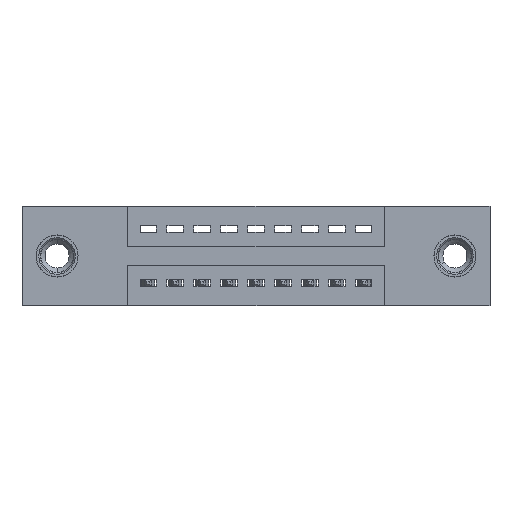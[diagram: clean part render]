
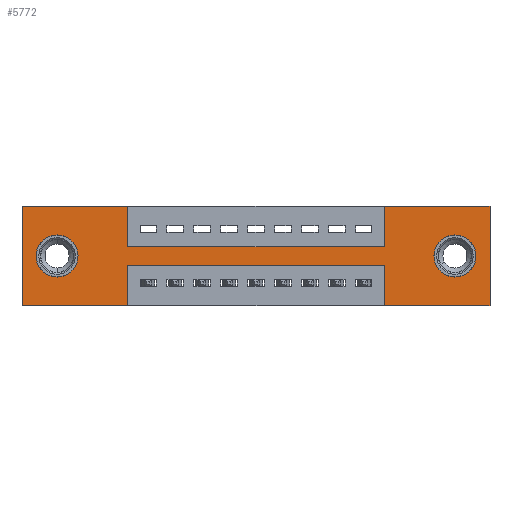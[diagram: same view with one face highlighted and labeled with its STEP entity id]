
A CAD part, front view. The second image highlights one B-rep face of the part: STEP entity #5772.
In plain terms, the highlighted planar face has unit normal (0, -1, 0).
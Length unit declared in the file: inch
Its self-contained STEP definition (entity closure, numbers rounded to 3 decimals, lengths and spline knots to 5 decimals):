
#291 = VERTEX_POINT ( 'NONE', #11541 ) ;
#350 = ORIENTED_EDGE ( 'NONE', *, *, #7089, .F. ) ;
#595 = ORIENTED_EDGE ( 'NONE', *, *, #1682, .F. ) ;
#609 = AXIS2_PLACEMENT_3D ( 'NONE', #12363, #6774, #968 ) ;
#776 = ORIENTED_EDGE ( 'NONE', *, *, #9528, .F. ) ;
#789 = CARTESIAN_POINT ( 'NONE',  ( 0., 0., 0. ) ) ;
#835 = ORIENTED_EDGE ( 'NONE', *, *, #6167, .T. ) ;
#839 = LINE ( 'NONE', #3806, #8551 ) ;
#843 = VECTOR ( 'NONE', #8535, 39.37008 ) ;
#883 = CARTESIAN_POINT ( 'NONE',  ( 1.3425, 0., 0. ) ) ;
#905 = LINE ( 'NONE', #2048, #5767 ) ;
#967 = EDGE_CURVE ( 'NONE', #3909, #5645, #2659, .T. ) ;
#968 = DIRECTION ( 'NONE',  ( 0., 0., 1. ) ) ;
#1172 = DIRECTION ( 'NONE',  ( 0., 0., -1. ) ) ;
#1248 = AXIS2_PLACEMENT_3D ( 'NONE', #11172, #5536, #12098 ) ;
#1309 = VERTEX_POINT ( 'NONE', #11852 ) ;
#1364 = CARTESIAN_POINT ( 'NONE',  ( 1.3425, 0., -0.37 ) ) ;
#1485 = VERTEX_POINT ( 'NONE', #883 ) ;
#1540 = EDGE_CURVE ( 'NONE', #4583, #1983, #10960, .T. ) ;
#1682 = EDGE_CURVE ( 'NONE', #1485, #10315, #11670, .T. ) ;
#1812 = VECTOR ( 'NONE', #2755, 39.37008 ) ;
#1960 = CARTESIAN_POINT ( 'NONE',  ( 0.3925, 0., 0. ) ) ;
#1983 = VERTEX_POINT ( 'NONE', #8934 ) ;
#2048 = CARTESIAN_POINT ( 'NONE',  ( 0.3925, 0., -0.15 ) ) ;
#2102 = VECTOR ( 'NONE', #9340, 39.37008 ) ;
#2384 = ORIENTED_EDGE ( 'NONE', *, *, #7300, .T. ) ;
#2472 = CARTESIAN_POINT ( 'NONE',  ( 0.3925, 0., -0.22 ) ) ;
#2659 = CIRCLE ( 'NONE', #7016, 0.078 ) ;
#2755 = DIRECTION ( 'NONE',  ( -1., 0., 0. ) ) ;
#2820 = EDGE_CURVE ( 'NONE', #4126, #1309, #3379, .T. ) ;
#2855 = LINE ( 'NONE', #1960, #7664 ) ;
#2918 = CARTESIAN_POINT ( 'NONE',  ( 0.13, 0., -0.107 ) ) ;
#2984 = EDGE_CURVE ( 'NONE', #9072, #1485, #9177, .T. ) ;
#3079 = VERTEX_POINT ( 'NONE', #8662 ) ;
#3239 = ORIENTED_EDGE ( 'NONE', *, *, #5587, .F. ) ;
#3243 = VERTEX_POINT ( 'NONE', #1364 ) ;
#3330 = DIRECTION ( 'NONE',  ( 0., 0., -1. ) ) ;
#3379 = CIRCLE ( 'NONE', #7757, 0.078 ) ;
#3417 = VECTOR ( 'NONE', #7366, 39.37008 ) ;
#3422 = EDGE_CURVE ( 'NONE', #10061, #3079, #9454, .T. ) ;
#3432 = CIRCLE ( 'NONE', #1248, 0.078 ) ;
#3484 = LINE ( 'NONE', #11287, #843 ) ;
#3499 = EDGE_CURVE ( 'NONE', #3079, #291, #8580, .T. ) ;
#3501 = DIRECTION ( 'NONE',  ( 0., 1., 0. ) ) ;
#3519 = VECTOR ( 'NONE', #7538, 39.37008 ) ;
#3806 = CARTESIAN_POINT ( 'NONE',  ( 0., 0., -0.37 ) ) ;
#3848 = DIRECTION ( 'NONE',  ( 0., 0., -1. ) ) ;
#3909 = VERTEX_POINT ( 'NONE', #9100 ) ;
#3915 = FACE_BOUND ( 'NONE', #11720, .T. ) ;
#3995 = DIRECTION ( 'NONE',  ( 1., 0., 0. ) ) ;
#4126 = VERTEX_POINT ( 'NONE', #12198 ) ;
#4287 = CARTESIAN_POINT ( 'NONE',  ( 1.735, 0., 0. ) ) ;
#4409 = VECTOR ( 'NONE', #9259, 39.37008 ) ;
#4583 = VERTEX_POINT ( 'NONE', #5063 ) ;
#4952 = ORIENTED_EDGE ( 'NONE', *, *, #2820, .T. ) ;
#5037 = PLANE ( 'NONE',  #9493 ) ;
#5063 = CARTESIAN_POINT ( 'NONE',  ( 1.3425, 0., -0.22 ) ) ;
#5075 = ORIENTED_EDGE ( 'NONE', *, *, #2984, .F. ) ;
#5178 = DIRECTION ( 'NONE',  ( 0., 1., 0. ) ) ;
#5480 = CARTESIAN_POINT ( 'NONE',  ( 1.3425, 0., -0.15 ) ) ;
#5482 = EDGE_CURVE ( 'NONE', #1983, #12427, #7516, .T. ) ;
#5533 = CARTESIAN_POINT ( 'NONE',  ( 0.3925, 0., -0.37 ) ) ;
#5536 = DIRECTION ( 'NONE',  ( 0., 1., 0. ) ) ;
#5587 = EDGE_CURVE ( 'NONE', #12329, #3243, #839, .T. ) ;
#5643 = EDGE_CURVE ( 'NONE', #291, #11051, #2855, .T. ) ;
#5645 = VERTEX_POINT ( 'NONE', #2918 ) ;
#5767 = VECTOR ( 'NONE', #3995, 39.37008 ) ;
#5772 = ADVANCED_FACE ( 'NONE', ( #11153, #3915, #6476 ), #5037, .T. ) ;
#5943 = CARTESIAN_POINT ( 'NONE',  ( 0., 0., -0.37 ) ) ;
#6167 = EDGE_CURVE ( 'NONE', #5645, #3909, #6460, .T. ) ;
#6460 = CIRCLE ( 'NONE', #609, 0.078 ) ;
#6476 = FACE_OUTER_BOUND ( 'NONE', #9864, .T. ) ;
#6579 = CARTESIAN_POINT ( 'NONE',  ( 0., 0., 0. ) ) ;
#6580 = ORIENTED_EDGE ( 'NONE', *, *, #3422, .F. ) ;
#6774 = DIRECTION ( 'NONE',  ( 0., 1., 0. ) ) ;
#6942 = DIRECTION ( 'NONE',  ( 0., -1., 0. ) ) ;
#7016 = AXIS2_PLACEMENT_3D ( 'NONE', #11821, #5178, #11853 ) ;
#7089 = EDGE_CURVE ( 'NONE', #10315, #12329, #8656, .T. ) ;
#7236 = CARTESIAN_POINT ( 'NONE',  ( 1.735, 0., -0.37 ) ) ;
#7300 = EDGE_CURVE ( 'NONE', #1309, #4126, #3432, .T. ) ;
#7366 = DIRECTION ( 'NONE',  ( -1., 0., 0. ) ) ;
#7516 = LINE ( 'NONE', #5533, #2102 ) ;
#7538 = DIRECTION ( 'NONE',  ( 1., 0., 0. ) ) ;
#7572 = DIRECTION ( 'NONE',  ( 1., 0., 0. ) ) ;
#7664 = VECTOR ( 'NONE', #3848, 39.37008 ) ;
#7757 = AXIS2_PLACEMENT_3D ( 'NONE', #9188, #3501, #10126 ) ;
#8372 = CARTESIAN_POINT ( 'NONE',  ( 0., 0., 0. ) ) ;
#8399 = EDGE_LOOP ( 'NONE', ( #2384, #4952 ) ) ;
#8501 = DIRECTION ( 'NONE',  ( 0., 0., 1. ) ) ;
#8535 = DIRECTION ( 'NONE',  ( 0., 0., 1. ) ) ;
#8551 = VECTOR ( 'NONE', #10426, 39.37008 ) ;
#8580 = LINE ( 'NONE', #6579, #3519 ) ;
#8607 = CARTESIAN_POINT ( 'NONE',  ( 0., 0., -0.37 ) ) ;
#8656 = LINE ( 'NONE', #4287, #11125 ) ;
#8662 = CARTESIAN_POINT ( 'NONE',  ( 0., 0., 0. ) ) ;
#8720 = ORIENTED_EDGE ( 'NONE', *, *, #11927, .F. ) ;
#8817 = CARTESIAN_POINT ( 'NONE',  ( 1.735, 0., 0. ) ) ;
#8854 = LINE ( 'NONE', #9425, #1812 ) ;
#8896 = VECTOR ( 'NONE', #8501, 39.37008 ) ;
#8934 = CARTESIAN_POINT ( 'NONE',  ( 0.3925, 0., -0.22 ) ) ;
#9072 = VERTEX_POINT ( 'NONE', #5480 ) ;
#9100 = CARTESIAN_POINT ( 'NONE',  ( 0.13, 0., -0.263 ) ) ;
#9129 = CARTESIAN_POINT ( 'NONE',  ( 0.3925, 0., -0.15 ) ) ;
#9177 = LINE ( 'NONE', #11247, #8896 ) ;
#9188 = CARTESIAN_POINT ( 'NONE',  ( 1.605, 0., -0.185 ) ) ;
#9259 = DIRECTION ( 'NONE',  ( 0., 0., 1. ) ) ;
#9340 = DIRECTION ( 'NONE',  ( 0., 0., -1. ) ) ;
#9425 = CARTESIAN_POINT ( 'NONE',  ( 0., 0., -0.37 ) ) ;
#9454 = LINE ( 'NONE', #8372, #4409 ) ;
#9493 = AXIS2_PLACEMENT_3D ( 'NONE', #5943, #6942, #1172 ) ;
#9528 = EDGE_CURVE ( 'NONE', #11051, #9072, #905, .T. ) ;
#9847 = ORIENTED_EDGE ( 'NONE', *, *, #11904, .F. ) ;
#9864 = EDGE_LOOP ( 'NONE', ( #11076, #10037, #8720, #3239, #350, #595, #5075, #776, #11135, #11564, #6580, #9847 ) ) ;
#10003 = ORIENTED_EDGE ( 'NONE', *, *, #967, .T. ) ;
#10037 = ORIENTED_EDGE ( 'NONE', *, *, #1540, .F. ) ;
#10061 = VERTEX_POINT ( 'NONE', #8607 ) ;
#10126 = DIRECTION ( 'NONE',  ( 0., 0., -1. ) ) ;
#10221 = CARTESIAN_POINT ( 'NONE',  ( 0.3925, 0., -0.37 ) ) ;
#10315 = VERTEX_POINT ( 'NONE', #8817 ) ;
#10426 = DIRECTION ( 'NONE',  ( -1., 0., 0. ) ) ;
#10960 = LINE ( 'NONE', #2472, #3417 ) ;
#11051 = VERTEX_POINT ( 'NONE', #9129 ) ;
#11076 = ORIENTED_EDGE ( 'NONE', *, *, #5482, .F. ) ;
#11125 = VECTOR ( 'NONE', #3330, 39.37008 ) ;
#11135 = ORIENTED_EDGE ( 'NONE', *, *, #5643, .F. ) ;
#11153 = FACE_BOUND ( 'NONE', #8399, .T. ) ;
#11172 = CARTESIAN_POINT ( 'NONE',  ( 1.605, 0., -0.185 ) ) ;
#11247 = CARTESIAN_POINT ( 'NONE',  ( 1.3425, 0., 0. ) ) ;
#11287 = CARTESIAN_POINT ( 'NONE',  ( 1.3425, 0., -0.37 ) ) ;
#11541 = CARTESIAN_POINT ( 'NONE',  ( 0.3925, 0., 0. ) ) ;
#11564 = ORIENTED_EDGE ( 'NONE', *, *, #3499, .F. ) ;
#11670 = LINE ( 'NONE', #789, #11966 ) ;
#11720 = EDGE_LOOP ( 'NONE', ( #835, #10003 ) ) ;
#11821 = CARTESIAN_POINT ( 'NONE',  ( 0.13, 0., -0.185 ) ) ;
#11852 = CARTESIAN_POINT ( 'NONE',  ( 1.605, 0., -0.107 ) ) ;
#11853 = DIRECTION ( 'NONE',  ( 0., 0., 1. ) ) ;
#11904 = EDGE_CURVE ( 'NONE', #12427, #10061, #8854, .T. ) ;
#11927 = EDGE_CURVE ( 'NONE', #3243, #4583, #3484, .T. ) ;
#11966 = VECTOR ( 'NONE', #7572, 39.37008 ) ;
#12098 = DIRECTION ( 'NONE',  ( 0., 0., -1. ) ) ;
#12198 = CARTESIAN_POINT ( 'NONE',  ( 1.605, 0., -0.263 ) ) ;
#12329 = VERTEX_POINT ( 'NONE', #7236 ) ;
#12363 = CARTESIAN_POINT ( 'NONE',  ( 0.13, 0., -0.185 ) ) ;
#12427 = VERTEX_POINT ( 'NONE', #10221 ) ;
